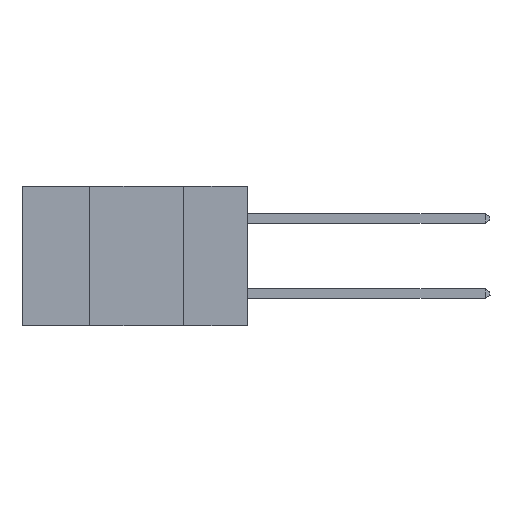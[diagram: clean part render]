
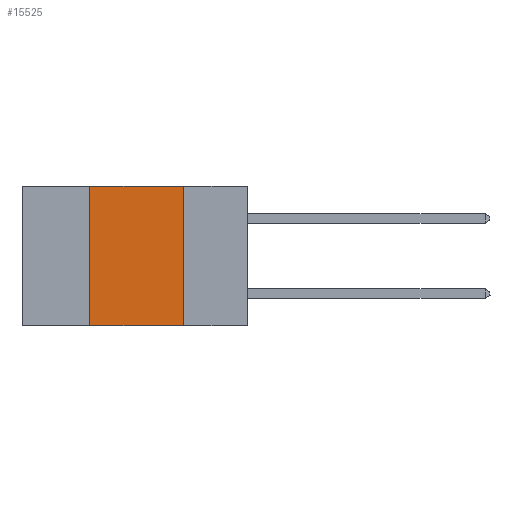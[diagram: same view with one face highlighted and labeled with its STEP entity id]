
A CAD part, left-side view. The second image highlights one B-rep face of the part: STEP entity #15525.
In plain terms, the highlighted planar face has unit normal (-1, 0, 0).
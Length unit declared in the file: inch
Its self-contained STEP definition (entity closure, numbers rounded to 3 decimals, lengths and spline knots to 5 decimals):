
#364 = CARTESIAN_POINT ( 'NONE',  ( 0., 0.17, 0. ) ) ;
#572 = VERTEX_POINT ( 'NONE', #11035 ) ;
#1784 = VECTOR ( 'NONE', #6265, 39.37008 ) ;
#2626 = CARTESIAN_POINT ( 'NONE',  ( 0., 0.42, -0.37 ) ) ;
#2765 = LINE ( 'NONE', #12914, #31291 ) ;
#2961 = LINE ( 'NONE', #11868, #1784 ) ;
#4141 = CARTESIAN_POINT ( 'NONE',  ( 0., 0.6, 0. ) ) ;
#6265 = DIRECTION ( 'NONE',  ( 0., -1., 0. ) ) ;
#7215 = VECTOR ( 'NONE', #30897, 39.37008 ) ;
#11035 = CARTESIAN_POINT ( 'NONE',  ( 0., 0.17, 0. ) ) ;
#11868 = CARTESIAN_POINT ( 'NONE',  ( 0., 0.6, -0.37 ) ) ;
#12690 = DIRECTION ( 'NONE',  ( 0., -1., 0. ) ) ;
#12761 = EDGE_CURVE ( 'NONE', #33064, #572, #2765, .T. ) ;
#12914 = CARTESIAN_POINT ( 'NONE',  ( 0., 0.6, 0. ) ) ;
#13795 = EDGE_CURVE ( 'NONE', #32328, #33064, #23347, .T. ) ;
#15525 = ADVANCED_FACE ( 'NONE', ( #15569 ), #16210, .F. ) ;
#15569 = FACE_OUTER_BOUND ( 'NONE', #25859, .T. ) ;
#16210 = PLANE ( 'NONE',  #31066 ) ;
#16765 = DIRECTION ( 'NONE',  ( 0., 0., -1. ) ) ;
#17343 = EDGE_CURVE ( 'NONE', #32328, #18010, #2961, .T. ) ;
#18010 = VERTEX_POINT ( 'NONE', #28965 ) ;
#20489 = VECTOR ( 'NONE', #32319, 39.37008 ) ;
#23347 = LINE ( 'NONE', #27175, #20489 ) ;
#24501 = LINE ( 'NONE', #364, #7215 ) ;
#24714 = DIRECTION ( 'NONE',  ( 1., 0., 0. ) ) ;
#25859 = EDGE_LOOP ( 'NONE', ( #29452, #26419, #27388, #31548 ) ) ;
#26419 = ORIENTED_EDGE ( 'NONE', *, *, #12761, .F. ) ;
#27175 = CARTESIAN_POINT ( 'NONE',  ( 0., 0.42, 0. ) ) ;
#27388 = ORIENTED_EDGE ( 'NONE', *, *, #13795, .F. ) ;
#28965 = CARTESIAN_POINT ( 'NONE',  ( 0., 0.17, -0.37 ) ) ;
#29452 = ORIENTED_EDGE ( 'NONE', *, *, #31568, .F. ) ;
#30897 = DIRECTION ( 'NONE',  ( 0., 0., -1. ) ) ;
#31066 = AXIS2_PLACEMENT_3D ( 'NONE', #4141, #24714, #16765 ) ;
#31291 = VECTOR ( 'NONE', #12690, 39.37008 ) ;
#31548 = ORIENTED_EDGE ( 'NONE', *, *, #17343, .T. ) ;
#31568 = EDGE_CURVE ( 'NONE', #572, #18010, #24501, .T. ) ;
#31668 = CARTESIAN_POINT ( 'NONE',  ( 0., 0.42, 0. ) ) ;
#32319 = DIRECTION ( 'NONE',  ( 0., 0., 1. ) ) ;
#32328 = VERTEX_POINT ( 'NONE', #2626 ) ;
#33064 = VERTEX_POINT ( 'NONE', #31668 ) ;
